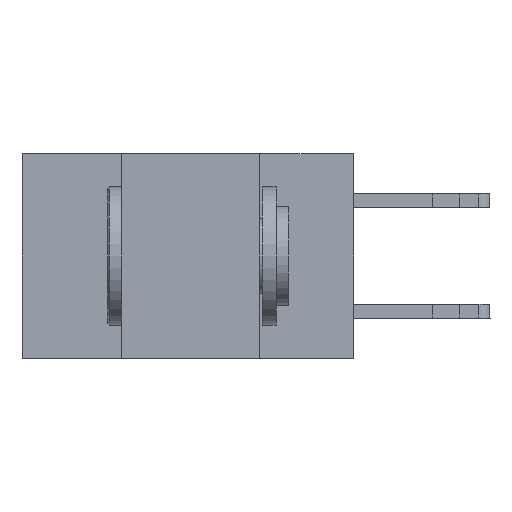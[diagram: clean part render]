
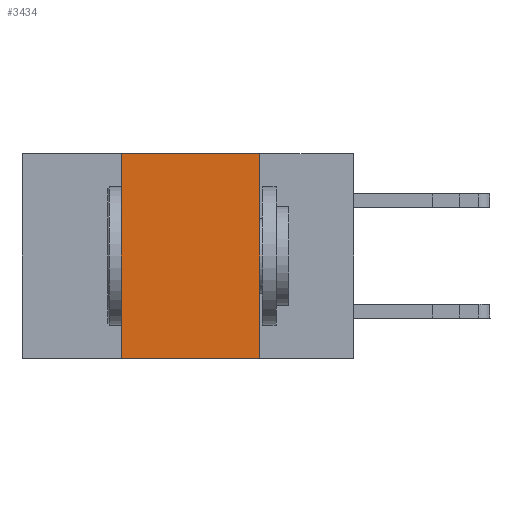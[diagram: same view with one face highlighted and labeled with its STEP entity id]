
A CAD part, left-side view. The second image highlights one B-rep face of the part: STEP entity #3434.
In plain terms, the highlighted planar face has unit normal (-1, 0, 0).
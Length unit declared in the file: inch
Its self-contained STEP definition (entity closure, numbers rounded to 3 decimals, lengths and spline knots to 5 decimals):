
#1108 = LINE ( 'NONE', #17019, #7248 ) ;
#1479 = LINE ( 'NONE', #20015, #19090 ) ;
#1825 = DIRECTION ( 'NONE',  ( 0., -1., 0. ) ) ;
#2005 = DIRECTION ( 'NONE',  ( 1., 0., 0. ) ) ;
#2962 = DIRECTION ( 'NONE',  ( 0., 0., 1. ) ) ;
#3434 = ADVANCED_FACE ( 'NONE', ( #28935 ), #13516, .F. ) ;
#4208 = DIRECTION ( 'NONE',  ( 0., -1., 0. ) ) ;
#5132 = EDGE_CURVE ( 'NONE', #9468, #18464, #10080, .T. ) ;
#7248 = VECTOR ( 'NONE', #2962, 39.37008 ) ;
#8075 = CARTESIAN_POINT ( 'NONE',  ( 0., 0.42, 0. ) ) ;
#8546 = ORIENTED_EDGE ( 'NONE', *, *, #22042, .F. ) ;
#8670 = VECTOR ( 'NONE', #1825, 39.37008 ) ;
#8797 = EDGE_LOOP ( 'NONE', ( #23030, #8546, #10304, #19080 ) ) ;
#9468 = VERTEX_POINT ( 'NONE', #11694 ) ;
#10080 = LINE ( 'NONE', #11186, #8670 ) ;
#10304 = ORIENTED_EDGE ( 'NONE', *, *, #17215, .F. ) ;
#11186 = CARTESIAN_POINT ( 'NONE',  ( 0., 0.6, -0.37 ) ) ;
#11618 = LINE ( 'NONE', #22910, #25311 ) ;
#11694 = CARTESIAN_POINT ( 'NONE',  ( 0., 0.42, -0.37 ) ) ;
#12509 = VERTEX_POINT ( 'NONE', #29512 ) ;
#13516 = PLANE ( 'NONE',  #24837 ) ;
#15793 = CARTESIAN_POINT ( 'NONE',  ( 0., 0.6, 0. ) ) ;
#16597 = VERTEX_POINT ( 'NONE', #8075 ) ;
#17019 = CARTESIAN_POINT ( 'NONE',  ( 0., 0.42, 0. ) ) ;
#17215 = EDGE_CURVE ( 'NONE', #9468, #16597, #1108, .T. ) ;
#18464 = VERTEX_POINT ( 'NONE', #26902 ) ;
#18485 = EDGE_CURVE ( 'NONE', #12509, #18464, #1479, .T. ) ;
#19080 = ORIENTED_EDGE ( 'NONE', *, *, #5132, .T. ) ;
#19090 = VECTOR ( 'NONE', #24354, 39.37008 ) ;
#20015 = CARTESIAN_POINT ( 'NONE',  ( 0., 0.17, 0. ) ) ;
#22042 = EDGE_CURVE ( 'NONE', #16597, #12509, #11618, .T. ) ;
#22910 = CARTESIAN_POINT ( 'NONE',  ( 0., 0.6, 0. ) ) ;
#23030 = ORIENTED_EDGE ( 'NONE', *, *, #18485, .F. ) ;
#24354 = DIRECTION ( 'NONE',  ( 0., 0., -1. ) ) ;
#24837 = AXIS2_PLACEMENT_3D ( 'NONE', #15793, #2005, #27398 ) ;
#25311 = VECTOR ( 'NONE', #4208, 39.37008 ) ;
#26902 = CARTESIAN_POINT ( 'NONE',  ( 0., 0.17, -0.37 ) ) ;
#27398 = DIRECTION ( 'NONE',  ( 0., 0., -1. ) ) ;
#28935 = FACE_OUTER_BOUND ( 'NONE', #8797, .T. ) ;
#29512 = CARTESIAN_POINT ( 'NONE',  ( 0., 0.17, 0. ) ) ;
